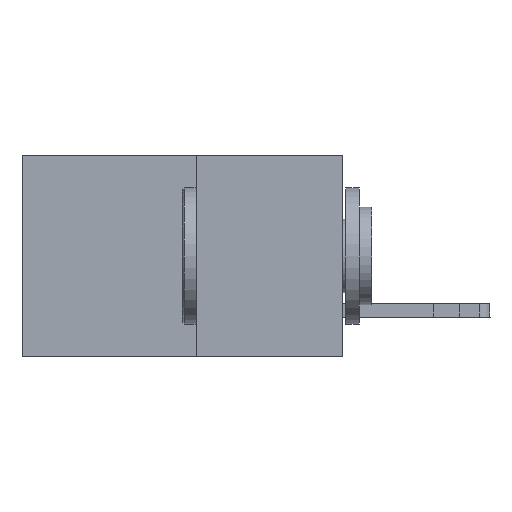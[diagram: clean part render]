
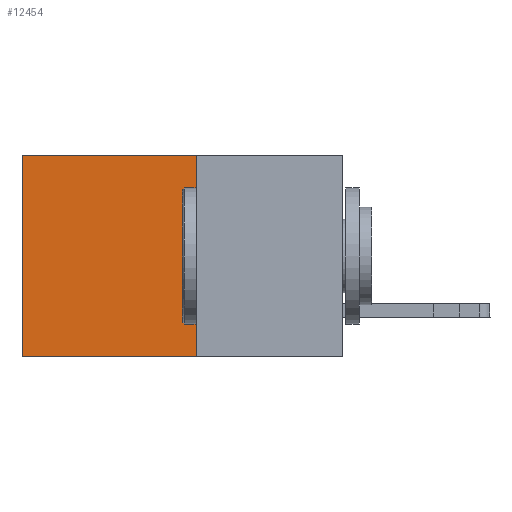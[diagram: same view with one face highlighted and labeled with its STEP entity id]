
A CAD part, left-side view. The second image highlights one B-rep face of the part: STEP entity #12454.
In plain terms, the highlighted planar face has unit normal (-1, 0, 0).
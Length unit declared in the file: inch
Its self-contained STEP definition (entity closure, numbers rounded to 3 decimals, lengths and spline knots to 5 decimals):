
#548 = VERTEX_POINT ( 'NONE', #6808 ) ;
#630 = PLANE ( 'NONE',  #13321 ) ;
#1817 = DIRECTION ( 'NONE',  ( 0., 0., -1. ) ) ;
#1983 = ORIENTED_EDGE ( 'NONE', *, *, #11273, .T. ) ;
#2537 = EDGE_CURVE ( 'NONE', #548, #13055, #6298, .T. ) ;
#2859 = VECTOR ( 'NONE', #1817, 39.37008 ) ;
#2911 = DIRECTION ( 'NONE',  ( 0., 1., 0. ) ) ;
#3613 = CARTESIAN_POINT ( 'NONE',  ( 0.277, 0.27, 0. ) ) ;
#3646 = ORIENTED_EDGE ( 'NONE', *, *, #4306, .F. ) ;
#3859 = CARTESIAN_POINT ( 'NONE',  ( 0.277, 0.59, -0.37 ) ) ;
#3939 = EDGE_LOOP ( 'NONE', ( #7736, #3646, #9157, #1983 ) ) ;
#4306 = EDGE_CURVE ( 'NONE', #13055, #10429, #11514, .T. ) ;
#4888 = VECTOR ( 'NONE', #2911, 39.37008 ) ;
#5034 = VERTEX_POINT ( 'NONE', #11483 ) ;
#5886 = LINE ( 'NONE', #10386, #12013 ) ;
#6298 = LINE ( 'NONE', #11248, #2859 ) ;
#6808 = CARTESIAN_POINT ( 'NONE',  ( 0.277, 0.27, 0. ) ) ;
#6827 = CARTESIAN_POINT ( 'NONE',  ( 0.277, 0.27, -0.37 ) ) ;
#7736 = ORIENTED_EDGE ( 'NONE', *, *, #13212, .T. ) ;
#7805 = DIRECTION ( 'NONE',  ( 0., 1., 0. ) ) ;
#7999 = LINE ( 'NONE', #3613, #9556 ) ;
#8072 = CARTESIAN_POINT ( 'NONE',  ( 0.277, 0.27, -0.37 ) ) ;
#9157 = ORIENTED_EDGE ( 'NONE', *, *, #2537, .F. ) ;
#9215 = DIRECTION ( 'NONE',  ( 0., 0., -1. ) ) ;
#9556 = VECTOR ( 'NONE', #7805, 39.37008 ) ;
#10061 = FACE_OUTER_BOUND ( 'NONE', #3939, .T. ) ;
#10386 = CARTESIAN_POINT ( 'NONE',  ( 0.277, 0.59, -0.37 ) ) ;
#10429 = VERTEX_POINT ( 'NONE', #3859 ) ;
#11248 = CARTESIAN_POINT ( 'NONE',  ( 0.277, 0.27, -0.37 ) ) ;
#11273 = EDGE_CURVE ( 'NONE', #548, #5034, #7999, .T. ) ;
#11483 = CARTESIAN_POINT ( 'NONE',  ( 0.277, 0.59, 0. ) ) ;
#11514 = LINE ( 'NONE', #12329, #4888 ) ;
#12013 = VECTOR ( 'NONE', #9215, 39.37008 ) ;
#12329 = CARTESIAN_POINT ( 'NONE',  ( 0.277, 0.27, -0.37 ) ) ;
#12454 = ADVANCED_FACE ( 'NONE', ( #10061 ), #630, .F. ) ;
#13055 = VERTEX_POINT ( 'NONE', #6827 ) ;
#13099 = DIRECTION ( 'NONE',  ( 0., 0., -1. ) ) ;
#13212 = EDGE_CURVE ( 'NONE', #5034, #10429, #5886, .T. ) ;
#13302 = DIRECTION ( 'NONE',  ( 1., 0., 0. ) ) ;
#13321 = AXIS2_PLACEMENT_3D ( 'NONE', #8072, #13302, #13099 ) ;
